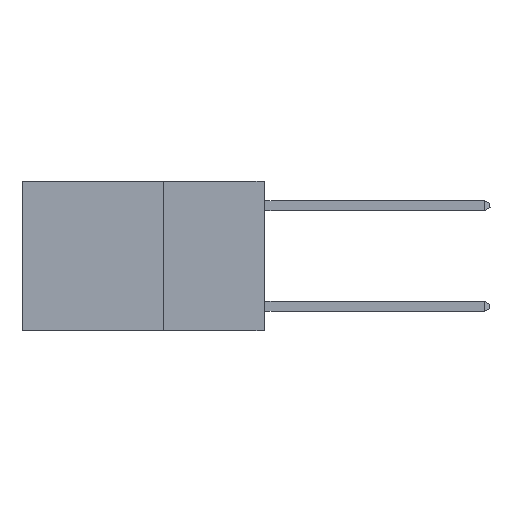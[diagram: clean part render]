
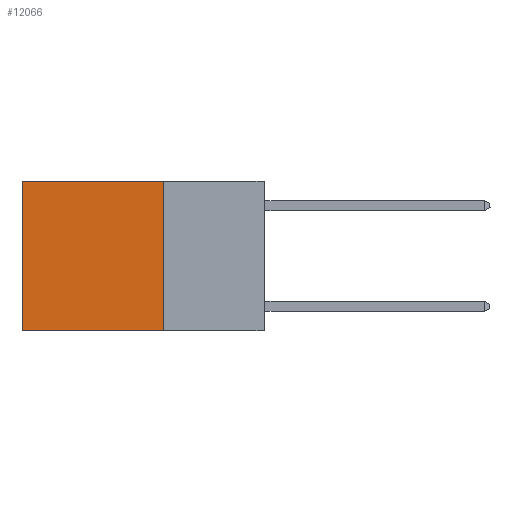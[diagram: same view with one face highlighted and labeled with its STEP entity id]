
A CAD part, left-side view. The second image highlights one B-rep face of the part: STEP entity #12066.
In plain terms, the highlighted planar face has unit normal (-1, 0, 0).
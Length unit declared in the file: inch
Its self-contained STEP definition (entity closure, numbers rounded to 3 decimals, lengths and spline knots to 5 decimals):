
#370 = ORIENTED_EDGE ( 'NONE', *, *, #2664, .T. ) ;
#575 = CARTESIAN_POINT ( 'NONE',  ( 0.2625, 0.25, 0. ) ) ;
#910 = EDGE_CURVE ( 'NONE', #5361, #18517, #8893, .T. ) ;
#2664 = EDGE_CURVE ( 'NONE', #18517, #12101, #9765, .T. ) ;
#3068 = CARTESIAN_POINT ( 'NONE',  ( 0.2625, 0.6, 0. ) ) ;
#3594 = DIRECTION ( 'NONE',  ( 0., 1., 0. ) ) ;
#5361 = VERTEX_POINT ( 'NONE', #575 ) ;
#5629 = VERTEX_POINT ( 'NONE', #7021 ) ;
#5939 = VECTOR ( 'NONE', #10501, 39.37008 ) ;
#6278 = CARTESIAN_POINT ( 'NONE',  ( 0.2625, 0.6, -0.37 ) ) ;
#6599 = VECTOR ( 'NONE', #6907, 39.37008 ) ;
#6907 = DIRECTION ( 'NONE',  ( 0., 0., -1. ) ) ;
#7021 = CARTESIAN_POINT ( 'NONE',  ( 0.2625, 0.25, -0.37 ) ) ;
#7868 = CARTESIAN_POINT ( 'NONE',  ( 0.2625, 0.25, 0. ) ) ;
#8348 = LINE ( 'NONE', #16120, #12015 ) ;
#8893 = LINE ( 'NONE', #7868, #9347 ) ;
#9347 = VECTOR ( 'NONE', #3594, 39.37008 ) ;
#9765 = LINE ( 'NONE', #18524, #6599 ) ;
#10501 = DIRECTION ( 'NONE',  ( 0., 0., -1. ) ) ;
#10629 = DIRECTION ( 'NONE',  ( 0., 0., -1. ) ) ;
#11638 = ORIENTED_EDGE ( 'NONE', *, *, #910, .T. ) ;
#11940 = EDGE_LOOP ( 'NONE', ( #370, #13957, #15464, #11638 ) ) ;
#12015 = VECTOR ( 'NONE', #17569, 39.37008 ) ;
#12031 = FACE_OUTER_BOUND ( 'NONE', #11940, .T. ) ;
#12066 = ADVANCED_FACE ( 'NONE', ( #12031 ), #13584, .F. ) ;
#12101 = VERTEX_POINT ( 'NONE', #6278 ) ;
#12261 = AXIS2_PLACEMENT_3D ( 'NONE', #16367, #17816, #10629 ) ;
#12440 = EDGE_CURVE ( 'NONE', #5629, #12101, #8348, .T. ) ;
#13460 = CARTESIAN_POINT ( 'NONE',  ( 0.2625, 0.25, 0. ) ) ;
#13584 = PLANE ( 'NONE',  #12261 ) ;
#13957 = ORIENTED_EDGE ( 'NONE', *, *, #12440, .F. ) ;
#14048 = LINE ( 'NONE', #13460, #5939 ) ;
#15464 = ORIENTED_EDGE ( 'NONE', *, *, #17347, .F. ) ;
#16120 = CARTESIAN_POINT ( 'NONE',  ( 0.2625, 0.25, -0.37 ) ) ;
#16367 = CARTESIAN_POINT ( 'NONE',  ( 0.2625, 0.25, 0. ) ) ;
#17347 = EDGE_CURVE ( 'NONE', #5361, #5629, #14048, .T. ) ;
#17569 = DIRECTION ( 'NONE',  ( 0., 1., 0. ) ) ;
#17816 = DIRECTION ( 'NONE',  ( 1., 0., 0. ) ) ;
#18517 = VERTEX_POINT ( 'NONE', #3068 ) ;
#18524 = CARTESIAN_POINT ( 'NONE',  ( 0.2625, 0.6, 0. ) ) ;
